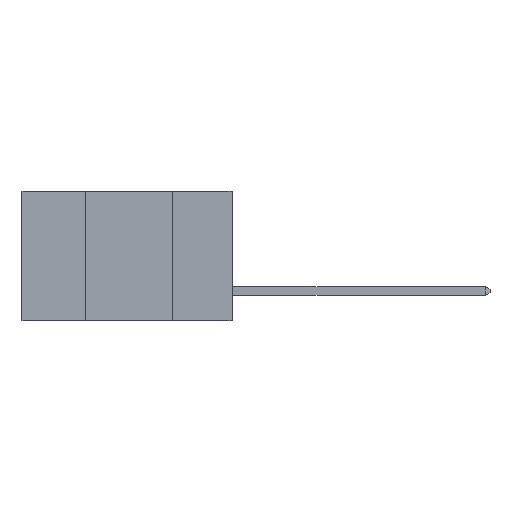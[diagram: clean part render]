
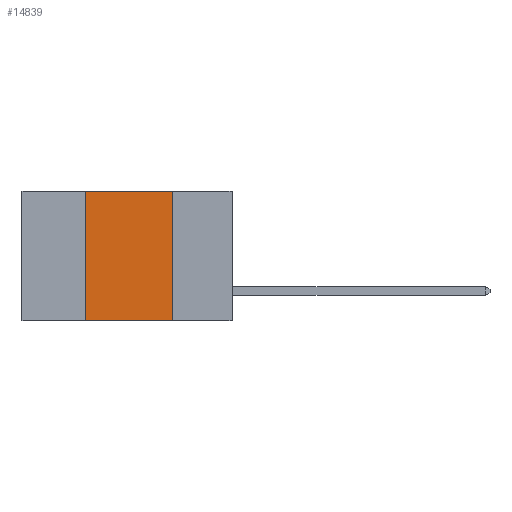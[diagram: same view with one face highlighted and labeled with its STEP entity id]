
A CAD part, left-side view. The second image highlights one B-rep face of the part: STEP entity #14839.
In plain terms, the highlighted planar face has unit normal (-1, 0, 0).
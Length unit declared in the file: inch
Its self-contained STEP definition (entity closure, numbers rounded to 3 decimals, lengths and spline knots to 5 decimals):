
#134 = LINE ( 'NONE', #12969, #10547 ) ;
#753 = VERTEX_POINT ( 'NONE', #17502 ) ;
#2029 = CARTESIAN_POINT ( 'NONE',  ( 0., 0.17, 0. ) ) ;
#2199 = VERTEX_POINT ( 'NONE', #9838 ) ;
#2719 = CARTESIAN_POINT ( 'NONE',  ( 0., 0.6, -0.37 ) ) ;
#3057 = DIRECTION ( 'NONE',  ( 0., 0., -1. ) ) ;
#3137 = ORIENTED_EDGE ( 'NONE', *, *, #22117, .F. ) ;
#3593 = VECTOR ( 'NONE', #20437, 39.37008 ) ;
#3932 = AXIS2_PLACEMENT_3D ( 'NONE', #13325, #15309, #3057 ) ;
#4767 = EDGE_LOOP ( 'NONE', ( #7637, #3137, #21871, #8707 ) ) ;
#4813 = DIRECTION ( 'NONE',  ( 0., -1., 0. ) ) ;
#4867 = LINE ( 'NONE', #19705, #9724 ) ;
#6918 = DIRECTION ( 'NONE',  ( 0., -1., 0. ) ) ;
#7637 = ORIENTED_EDGE ( 'NONE', *, *, #8945, .F. ) ;
#7640 = VERTEX_POINT ( 'NONE', #23750 ) ;
#7654 = DIRECTION ( 'NONE',  ( 0., 0., 1. ) ) ;
#8315 = VECTOR ( 'NONE', #6918, 39.37008 ) ;
#8416 = CARTESIAN_POINT ( 'NONE',  ( 0., 0.42, 0. ) ) ;
#8462 = LINE ( 'NONE', #2029, #3593 ) ;
#8707 = ORIENTED_EDGE ( 'NONE', *, *, #12204, .T. ) ;
#8945 = EDGE_CURVE ( 'NONE', #7640, #2199, #8462, .T. ) ;
#9724 = VECTOR ( 'NONE', #7654, 39.37008 ) ;
#9838 = CARTESIAN_POINT ( 'NONE',  ( 0., 0.17, -0.37 ) ) ;
#10547 = VECTOR ( 'NONE', #4813, 39.37008 ) ;
#12204 = EDGE_CURVE ( 'NONE', #753, #2199, #13731, .T. ) ;
#12969 = CARTESIAN_POINT ( 'NONE',  ( 0., 0.6, 0. ) ) ;
#13325 = CARTESIAN_POINT ( 'NONE',  ( 0., 0.6, 0. ) ) ;
#13731 = LINE ( 'NONE', #2719, #8315 ) ;
#14839 = ADVANCED_FACE ( 'NONE', ( #23673 ), #25140, .F. ) ;
#15309 = DIRECTION ( 'NONE',  ( 1., 0., 0. ) ) ;
#17502 = CARTESIAN_POINT ( 'NONE',  ( 0., 0.42, -0.37 ) ) ;
#19128 = EDGE_CURVE ( 'NONE', #753, #20012, #4867, .T. ) ;
#19705 = CARTESIAN_POINT ( 'NONE',  ( 0., 0.42, 0. ) ) ;
#20012 = VERTEX_POINT ( 'NONE', #8416 ) ;
#20437 = DIRECTION ( 'NONE',  ( 0., 0., -1. ) ) ;
#21871 = ORIENTED_EDGE ( 'NONE', *, *, #19128, .F. ) ;
#22117 = EDGE_CURVE ( 'NONE', #20012, #7640, #134, .T. ) ;
#23673 = FACE_OUTER_BOUND ( 'NONE', #4767, .T. ) ;
#23750 = CARTESIAN_POINT ( 'NONE',  ( 0., 0.17, 0. ) ) ;
#25140 = PLANE ( 'NONE',  #3932 ) ;
